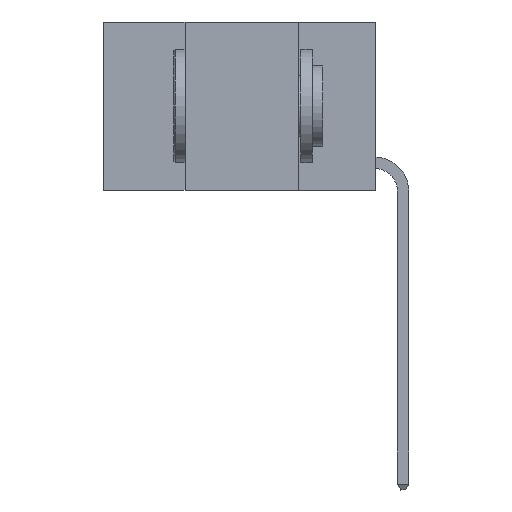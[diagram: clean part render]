
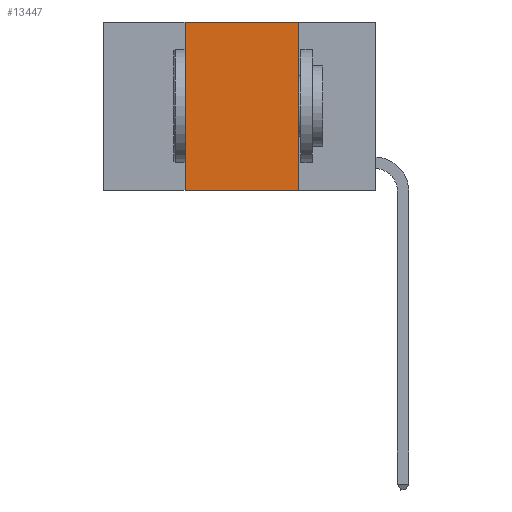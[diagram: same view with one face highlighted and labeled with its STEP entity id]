
A CAD part, left-side view. The second image highlights one B-rep face of the part: STEP entity #13447.
In plain terms, the highlighted planar face has unit normal (-1, 0, 0).
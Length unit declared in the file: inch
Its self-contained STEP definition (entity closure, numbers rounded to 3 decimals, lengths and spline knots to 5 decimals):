
#491 = EDGE_CURVE ( 'NONE', #3241, #13270, #24929, .T. ) ;
#615 = LINE ( 'NONE', #23625, #8875 ) ;
#1431 = EDGE_CURVE ( 'NONE', #8917, #13488, #20550, .T. ) ;
#1468 = EDGE_LOOP ( 'NONE', ( #23322, #18384, #6766, #13228 ) ) ;
#1781 = DIRECTION ( 'NONE',  ( 0., -1., 0. ) ) ;
#2531 = CARTESIAN_POINT ( 'NONE',  ( 0., 0.42, 0. ) ) ;
#3241 = VERTEX_POINT ( 'NONE', #22700 ) ;
#3440 = VECTOR ( 'NONE', #24972, 39.37008 ) ;
#3683 = FACE_OUTER_BOUND ( 'NONE', #1468, .T. ) ;
#3830 = CARTESIAN_POINT ( 'NONE',  ( 0., 0.17, 0. ) ) ;
#6766 = ORIENTED_EDGE ( 'NONE', *, *, #9445, .F. ) ;
#8875 = VECTOR ( 'NONE', #26068, 39.37008 ) ;
#8917 = VERTEX_POINT ( 'NONE', #2531 ) ;
#9445 = EDGE_CURVE ( 'NONE', #3241, #8917, #10780, .T. ) ;
#9704 = EDGE_CURVE ( 'NONE', #13488, #13270, #615, .T. ) ;
#10404 = VECTOR ( 'NONE', #1781, 39.37008 ) ;
#10780 = LINE ( 'NONE', #27160, #18179 ) ;
#13228 = ORIENTED_EDGE ( 'NONE', *, *, #491, .T. ) ;
#13270 = VERTEX_POINT ( 'NONE', #23791 ) ;
#13447 = ADVANCED_FACE ( 'NONE', ( #3683 ), #24841, .F. ) ;
#13488 = VERTEX_POINT ( 'NONE', #3830 ) ;
#17515 = DIRECTION ( 'NONE',  ( 0., 0., -1. ) ) ;
#18179 = VECTOR ( 'NONE', #24274, 39.37008 ) ;
#18384 = ORIENTED_EDGE ( 'NONE', *, *, #1431, .F. ) ;
#20550 = LINE ( 'NONE', #30008, #3440 ) ;
#20786 = AXIS2_PLACEMENT_3D ( 'NONE', #28973, #29122, #17515 ) ;
#22700 = CARTESIAN_POINT ( 'NONE',  ( 0., 0.42, -0.37 ) ) ;
#23322 = ORIENTED_EDGE ( 'NONE', *, *, #9704, .F. ) ;
#23625 = CARTESIAN_POINT ( 'NONE',  ( 0., 0.17, 0. ) ) ;
#23791 = CARTESIAN_POINT ( 'NONE',  ( 0., 0.17, -0.37 ) ) ;
#24274 = DIRECTION ( 'NONE',  ( 0., 0., 1. ) ) ;
#24841 = PLANE ( 'NONE',  #20786 ) ;
#24929 = LINE ( 'NONE', #29672, #10404 ) ;
#24972 = DIRECTION ( 'NONE',  ( 0., -1., 0. ) ) ;
#26068 = DIRECTION ( 'NONE',  ( 0., 0., -1. ) ) ;
#27160 = CARTESIAN_POINT ( 'NONE',  ( 0., 0.42, 0. ) ) ;
#28973 = CARTESIAN_POINT ( 'NONE',  ( 0., 0.6, 0. ) ) ;
#29122 = DIRECTION ( 'NONE',  ( 1., 0., 0. ) ) ;
#29672 = CARTESIAN_POINT ( 'NONE',  ( 0., 0.6, -0.37 ) ) ;
#30008 = CARTESIAN_POINT ( 'NONE',  ( 0., 0.6, 0. ) ) ;
